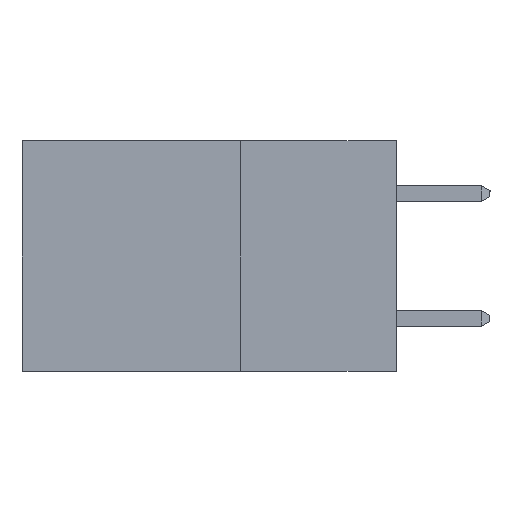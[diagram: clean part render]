
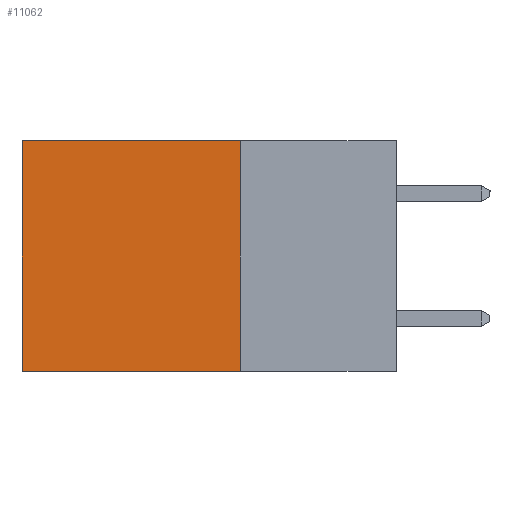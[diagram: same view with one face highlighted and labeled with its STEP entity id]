
A CAD part, left-side view. The second image highlights one B-rep face of the part: STEP entity #11062.
In plain terms, the highlighted planar face has unit normal (-1, 0, 0).
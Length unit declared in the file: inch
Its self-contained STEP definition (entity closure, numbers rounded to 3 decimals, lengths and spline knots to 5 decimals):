
#77 = EDGE_LOOP ( 'NONE', ( #5422, #1304, #3464, #8705 ) ) ;
#175 = CARTESIAN_POINT ( 'NONE',  ( 0.2615, 0.25, 0. ) ) ;
#283 = EDGE_CURVE ( 'NONE', #13913, #7732, #7000, .T. ) ;
#835 = CARTESIAN_POINT ( 'NONE',  ( 0.2615, 0.6, -0.37 ) ) ;
#1033 = CARTESIAN_POINT ( 'NONE',  ( 0.2615, 0.25, 0. ) ) ;
#1055 = DIRECTION ( 'NONE',  ( 0., 0., -1. ) ) ;
#1068 = VERTEX_POINT ( 'NONE', #1882 ) ;
#1304 = ORIENTED_EDGE ( 'NONE', *, *, #7107, .F. ) ;
#1882 = CARTESIAN_POINT ( 'NONE',  ( 0.2615, 0.6, 0. ) ) ;
#3251 = EDGE_CURVE ( 'NONE', #1068, #14576, #11398, .T. ) ;
#3430 = VECTOR ( 'NONE', #12313, 39.37008 ) ;
#3464 = ORIENTED_EDGE ( 'NONE', *, *, #283, .F. ) ;
#5216 = LINE ( 'NONE', #5295, #3430 ) ;
#5295 = CARTESIAN_POINT ( 'NONE',  ( 0.2615, 0.25, -0.37 ) ) ;
#5403 = DIRECTION ( 'NONE',  ( 0., 0., -1. ) ) ;
#5422 = ORIENTED_EDGE ( 'NONE', *, *, #3251, .T. ) ;
#5522 = DIRECTION ( 'NONE',  ( 0., 1., 0. ) ) ;
#5873 = CARTESIAN_POINT ( 'NONE',  ( 0.2615, 0.25, -0.37 ) ) ;
#6417 = CARTESIAN_POINT ( 'NONE',  ( 0.2615, 0.6, -0.37 ) ) ;
#7000 = LINE ( 'NONE', #11620, #9954 ) ;
#7107 = EDGE_CURVE ( 'NONE', #7732, #14576, #5216, .T. ) ;
#7216 = EDGE_CURVE ( 'NONE', #13913, #1068, #13914, .T. ) ;
#7732 = VERTEX_POINT ( 'NONE', #5873 ) ;
#8705 = ORIENTED_EDGE ( 'NONE', *, *, #7216, .T. ) ;
#9954 = VECTOR ( 'NONE', #1055, 39.37008 ) ;
#10431 = PLANE ( 'NONE',  #14203 ) ;
#10731 = DIRECTION ( 'NONE',  ( 0., 0., -1. ) ) ;
#10795 = VECTOR ( 'NONE', #5522, 39.37008 ) ;
#11062 = ADVANCED_FACE ( 'NONE', ( #11976 ), #10431, .F. ) ;
#11264 = VECTOR ( 'NONE', #5403, 39.37008 ) ;
#11398 = LINE ( 'NONE', #835, #11264 ) ;
#11620 = CARTESIAN_POINT ( 'NONE',  ( 0.2615, 0.25, -0.37 ) ) ;
#11815 = CARTESIAN_POINT ( 'NONE',  ( 0.2615, 0.25, -0.37 ) ) ;
#11976 = FACE_OUTER_BOUND ( 'NONE', #77, .T. ) ;
#12313 = DIRECTION ( 'NONE',  ( 0., 1., 0. ) ) ;
#13913 = VERTEX_POINT ( 'NONE', #175 ) ;
#13914 = LINE ( 'NONE', #1033, #10795 ) ;
#14203 = AXIS2_PLACEMENT_3D ( 'NONE', #11815, #15142, #10731 ) ;
#14576 = VERTEX_POINT ( 'NONE', #6417 ) ;
#15142 = DIRECTION ( 'NONE',  ( 1., 0., 0. ) ) ;
